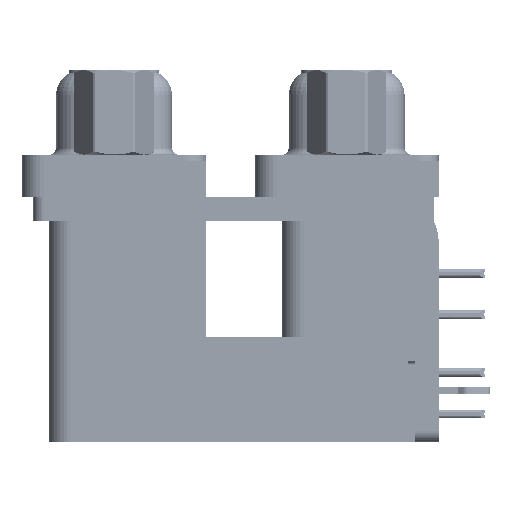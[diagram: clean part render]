
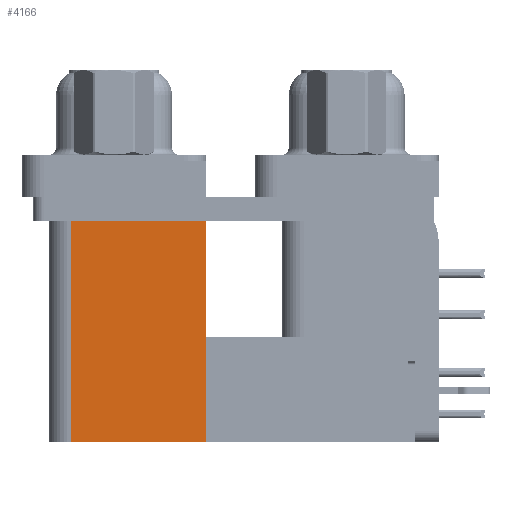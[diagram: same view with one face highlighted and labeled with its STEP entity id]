
A CAD part, left-side view. The second image highlights one B-rep face of the part: STEP entity #4166.
In plain terms, the highlighted planar face has unit normal (-1, 0, 0).
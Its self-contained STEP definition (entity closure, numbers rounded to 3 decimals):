
#2747 = CARTESIAN_POINT ( 'NONE',  ( 3.765, 9.6, -2.5 ) ) ;
#4067 = VERTEX_POINT ( 'NONE', #16199 ) ;
#4166 = ADVANCED_FACE ( 'NONE', ( #21255 ), #17028, .F. ) ;
#8607 = CARTESIAN_POINT ( 'NONE',  ( 3.765, 9.6, -19.2 ) ) ;
#9319 = VECTOR ( 'NONE', #37857, 1000. ) ;
#10860 = EDGE_CURVE ( 'NONE', #21747, #14317, #50760, .T. ) ;
#13558 = ORIENTED_EDGE ( 'NONE', *, *, #27895, .F. ) ;
#13662 = DIRECTION ( 'NONE',  ( 0., 0., -1. ) ) ;
#14317 = VERTEX_POINT ( 'NONE', #35542 ) ;
#16199 = CARTESIAN_POINT ( 'NONE',  ( 3.765, 18.8, -19.2 ) ) ;
#16615 = ORIENTED_EDGE ( 'NONE', *, *, #42769, .T. ) ;
#16820 = CARTESIAN_POINT ( 'NONE',  ( 3.765, 9.6, -2.5 ) ) ;
#17028 = PLANE ( 'NONE',  #40783 ) ;
#18721 = DIRECTION ( 'NONE',  ( 0., 0., 1. ) ) ;
#21255 = FACE_OUTER_BOUND ( 'NONE', #52615, .T. ) ;
#21747 = VERTEX_POINT ( 'NONE', #2747 ) ;
#22090 = DIRECTION ( 'NONE',  ( 1., 0., 0. ) ) ;
#23761 = LINE ( 'NONE', #48160, #49745 ) ;
#23918 = VECTOR ( 'NONE', #29576, 1000. ) ;
#27895 = EDGE_CURVE ( 'NONE', #28198, #4067, #30732, .T. ) ;
#28198 = VERTEX_POINT ( 'NONE', #53513 ) ;
#29576 = DIRECTION ( 'NONE',  ( 0., 0., 1. ) ) ;
#30635 = ORIENTED_EDGE ( 'NONE', *, *, #10860, .T. ) ;
#30732 = LINE ( 'NONE', #47828, #51110 ) ;
#35542 = CARTESIAN_POINT ( 'NONE',  ( 3.765, 18.8, -2.5 ) ) ;
#36676 = EDGE_CURVE ( 'NONE', #4067, #14317, #23761, .T. ) ;
#37430 = LINE ( 'NONE', #48001, #23918 ) ;
#37857 = DIRECTION ( 'NONE',  ( 0., 1., 0. ) ) ;
#39684 = DIRECTION ( 'NONE',  ( 0., 1., 0. ) ) ;
#40783 = AXIS2_PLACEMENT_3D ( 'NONE', #8607, #22090, #13662 ) ;
#42769 = EDGE_CURVE ( 'NONE', #28198, #21747, #37430, .T. ) ;
#47093 = ORIENTED_EDGE ( 'NONE', *, *, #36676, .F. ) ;
#47828 = CARTESIAN_POINT ( 'NONE',  ( 3.765, 9.6, -19.2 ) ) ;
#48001 = CARTESIAN_POINT ( 'NONE',  ( 3.765, 9.6, -19.2 ) ) ;
#48160 = CARTESIAN_POINT ( 'NONE',  ( 3.765, 18.8, -19.2 ) ) ;
#49745 = VECTOR ( 'NONE', #18721, 1000. ) ;
#50760 = LINE ( 'NONE', #16820, #9319 ) ;
#51110 = VECTOR ( 'NONE', #39684, 1000. ) ;
#52615 = EDGE_LOOP ( 'NONE', ( #30635, #47093, #13558, #16615 ) ) ;
#53513 = CARTESIAN_POINT ( 'NONE',  ( 3.765, 9.6, -19.2 ) ) ;
